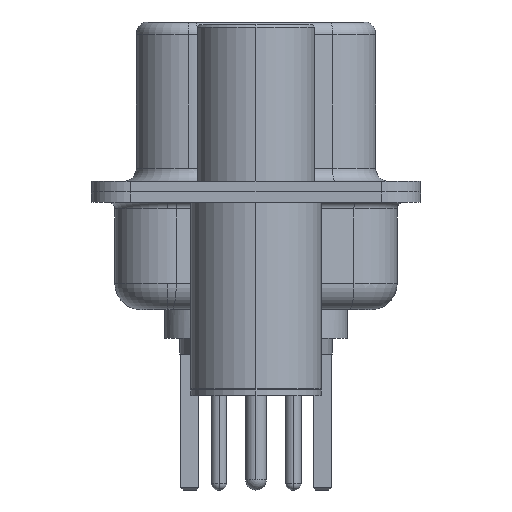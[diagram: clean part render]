
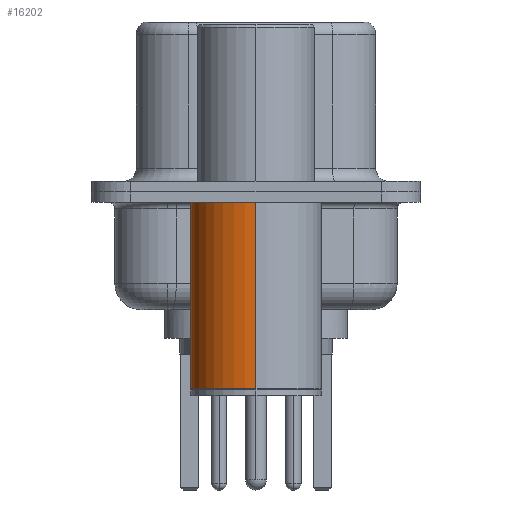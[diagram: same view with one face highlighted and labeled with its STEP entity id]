
A CAD part, left-side view. The second image highlights one B-rep face of the part: STEP entity #16202.
In plain terms, the highlighted cylindrical face has radius 2.5 mm (diameter 5 mm), a partial arc.
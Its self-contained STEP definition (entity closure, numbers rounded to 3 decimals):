
#2165 = DIRECTION ( 'NONE',  ( 0., 0., 1. ) ) ;
#2223 = DIRECTION ( 'NONE',  ( 0., 0., 1. ) ) ;
#2780 = VERTEX_POINT ( 'NONE', #13053 ) ;
#2815 = CARTESIAN_POINT ( 'NONE',  ( 0., 0., -7.525 ) ) ;
#3427 = EDGE_CURVE ( 'NONE', #4697, #2780, #10649, .T. ) ;
#3713 = CARTESIAN_POINT ( 'NONE',  ( -2.5, 0., -0.4 ) ) ;
#3762 = CARTESIAN_POINT ( 'NONE',  ( -2.5, 0., 0.581 ) ) ;
#4024 = VECTOR ( 'NONE', #5165, 1000. ) ;
#4697 = VERTEX_POINT ( 'NONE', #15542 ) ;
#4858 = CYLINDRICAL_SURFACE ( 'NONE', #6772, 2.5 ) ;
#5165 = DIRECTION ( 'NONE',  ( 0., 0., 1. ) ) ;
#5348 = FACE_OUTER_BOUND ( 'NONE', #18135, .T. ) ;
#5388 = CARTESIAN_POINT ( 'NONE',  ( 2.5, 0., -0.4 ) ) ;
#6494 = CIRCLE ( 'NONE', #18804, 2.5 ) ;
#6772 = AXIS2_PLACEMENT_3D ( 'NONE', #18460, #18522, #9278 ) ;
#7129 = EDGE_CURVE ( 'NONE', #4697, #9132, #8382, .T. ) ;
#8382 = LINE ( 'NONE', #9652, #4024 ) ;
#9132 = VERTEX_POINT ( 'NONE', #5388 ) ;
#9278 = DIRECTION ( 'NONE',  ( 1., 0., 0. ) ) ;
#9652 = CARTESIAN_POINT ( 'NONE',  ( 2.5, 0., 0.581 ) ) ;
#10152 = ORIENTED_EDGE ( 'NONE', *, *, #3427, .T. ) ;
#10649 = CIRCLE ( 'NONE', #14616, 2.5 ) ;
#11737 = CARTESIAN_POINT ( 'NONE',  ( 0., 0., -0.4 ) ) ;
#12272 = LINE ( 'NONE', #3762, #19476 ) ;
#13053 = CARTESIAN_POINT ( 'NONE',  ( -2.5, 0., -7.525 ) ) ;
#13293 = DIRECTION ( 'NONE',  ( 1., 0., 0. ) ) ;
#13829 = DIRECTION ( 'NONE',  ( 1., 0., 0. ) ) ;
#14375 = EDGE_CURVE ( 'NONE', #9132, #18802, #6494, .T. ) ;
#14616 = AXIS2_PLACEMENT_3D ( 'NONE', #2815, #15817, #13829 ) ;
#15542 = CARTESIAN_POINT ( 'NONE',  ( 2.5, 0., -7.525 ) ) ;
#15817 = DIRECTION ( 'NONE',  ( 0., 0., 1. ) ) ;
#16202 = ADVANCED_FACE ( 'NONE', ( #5348 ), #4858, .T. ) ;
#18135 = EDGE_LOOP ( 'NONE', ( #10152, #19455, #19859, #18685 ) ) ;
#18460 = CARTESIAN_POINT ( 'NONE',  ( 0., 0., 0.581 ) ) ;
#18522 = DIRECTION ( 'NONE',  ( 0., 0., 1. ) ) ;
#18685 = ORIENTED_EDGE ( 'NONE', *, *, #7129, .F. ) ;
#18802 = VERTEX_POINT ( 'NONE', #3713 ) ;
#18804 = AXIS2_PLACEMENT_3D ( 'NONE', #11737, #2223, #13293 ) ;
#19455 = ORIENTED_EDGE ( 'NONE', *, *, #19533, .T. ) ;
#19476 = VECTOR ( 'NONE', #2165, 1000. ) ;
#19533 = EDGE_CURVE ( 'NONE', #2780, #18802, #12272, .T. ) ;
#19859 = ORIENTED_EDGE ( 'NONE', *, *, #14375, .F. ) ;
